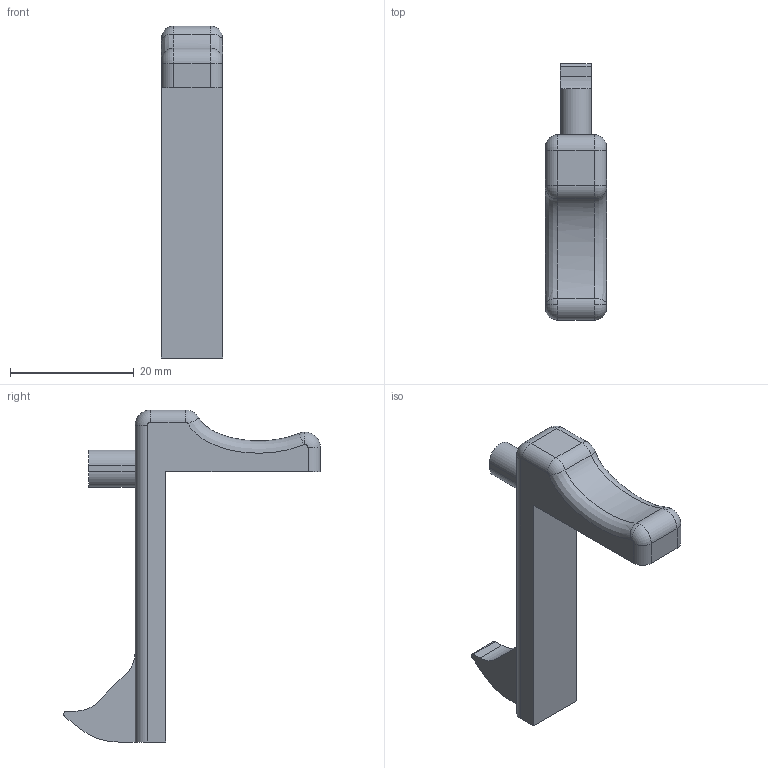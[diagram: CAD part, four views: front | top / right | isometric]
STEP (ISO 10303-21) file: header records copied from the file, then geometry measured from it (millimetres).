
FILE_DESCRIPTION (( 'STEP AP203' ), '1' );
FILE_NAME ('Trigger.STEP', '2013-11-14T05:08:54', ( '' ), ( '' ), 'SwSTEP 2.0', 'SolidWorks 2013', '' );
FILE_SCHEMA (( 'CONFIG_CONTROL_DESIGN' ));
Length unit declared in the file: millimetre
Products named in the file (1): Trigger
Bounding box: 9.9 x 41.57 x 53.75 mm (x, y, z)
Volume: 4696.6 mm3; surface area: 2683.2 mm2
Topology: 1 solids, 1 shells, 44 faces, 111 edges, 70 vertices
Faces by surface type: cylinder 17, plane 16, torus 8, bspline 3
Entity records: 1639 total; most frequent: CARTESIAN_POINT 479, DIRECTION 241, ORIENTED_EDGE 222, EDGE_CURVE 111, AXIS2_PLACEMENT_3D 92, VERTEX_POINT 70, VECTOR 57, LINE 57
